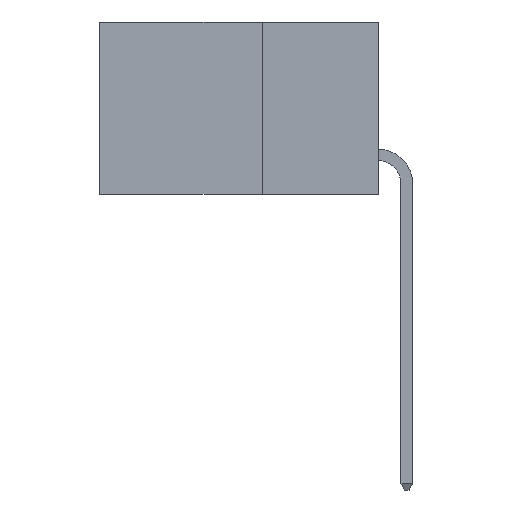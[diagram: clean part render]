
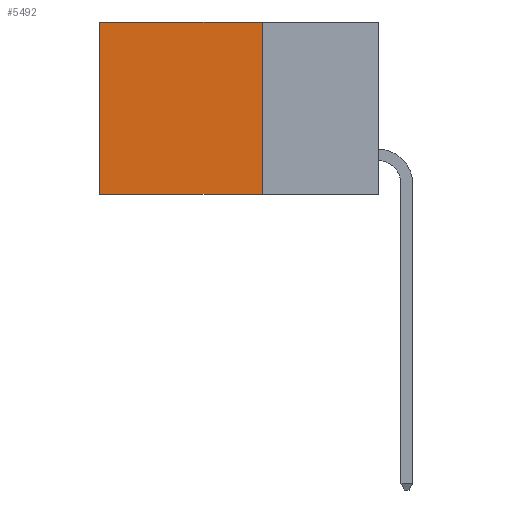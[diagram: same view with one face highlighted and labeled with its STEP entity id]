
A CAD part, left-side view. The second image highlights one B-rep face of the part: STEP entity #5492.
In plain terms, the highlighted planar face has unit normal (-1, 0, 0).
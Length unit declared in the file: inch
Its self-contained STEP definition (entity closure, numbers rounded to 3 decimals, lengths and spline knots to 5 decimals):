
#152 = PLANE ( 'NONE',  #8599 ) ;
#533 = LINE ( 'NONE', #5186, #8434 ) ;
#593 = CARTESIAN_POINT ( 'NONE',  ( 0.2615, 0.25, -0.37 ) ) ;
#1516 = VERTEX_POINT ( 'NONE', #2472 ) ;
#1662 = LINE ( 'NONE', #7751, #6808 ) ;
#1701 = CARTESIAN_POINT ( 'NONE',  ( 0.2615, 0.25, 0. ) ) ;
#1781 = VERTEX_POINT ( 'NONE', #12896 ) ;
#1804 = DIRECTION ( 'NONE',  ( 0., 0., -1. ) ) ;
#1983 = VECTOR ( 'NONE', #1804, 39.37008 ) ;
#2302 = LINE ( 'NONE', #3801, #1983 ) ;
#2472 = CARTESIAN_POINT ( 'NONE',  ( 0.2615, 0.6, -0.37 ) ) ;
#2528 = EDGE_CURVE ( 'NONE', #1781, #3534, #11298, .T. ) ;
#2982 = ORIENTED_EDGE ( 'NONE', *, *, #11586, .F. ) ;
#3303 = DIRECTION ( 'NONE',  ( 1., 0., 0. ) ) ;
#3534 = VERTEX_POINT ( 'NONE', #9424 ) ;
#3801 = CARTESIAN_POINT ( 'NONE',  ( 0.2615, 0.25, -0.37 ) ) ;
#4270 = EDGE_CURVE ( 'NONE', #9251, #1516, #1662, .T. ) ;
#4550 = ORIENTED_EDGE ( 'NONE', *, *, #4270, .F. ) ;
#5186 = CARTESIAN_POINT ( 'NONE',  ( 0.2615, 0.6, -0.37 ) ) ;
#5222 = EDGE_LOOP ( 'NONE', ( #5898, #4550, #2982, #10934 ) ) ;
#5492 = ADVANCED_FACE ( 'NONE', ( #10964 ), #152, .F. ) ;
#5898 = ORIENTED_EDGE ( 'NONE', *, *, #11180, .T. ) ;
#6808 = VECTOR ( 'NONE', #8762, 39.37008 ) ;
#7751 = CARTESIAN_POINT ( 'NONE',  ( 0.2615, 0.25, -0.37 ) ) ;
#7897 = DIRECTION ( 'NONE',  ( 0., 1., 0. ) ) ;
#8434 = VECTOR ( 'NONE', #12064, 39.37008 ) ;
#8599 = AXIS2_PLACEMENT_3D ( 'NONE', #9451, #3303, #10433 ) ;
#8762 = DIRECTION ( 'NONE',  ( 0., 1., 0. ) ) ;
#8772 = VECTOR ( 'NONE', #7897, 39.37008 ) ;
#9251 = VERTEX_POINT ( 'NONE', #593 ) ;
#9424 = CARTESIAN_POINT ( 'NONE',  ( 0.2615, 0.6, 0. ) ) ;
#9451 = CARTESIAN_POINT ( 'NONE',  ( 0.2615, 0.25, -0.37 ) ) ;
#10433 = DIRECTION ( 'NONE',  ( 0., 0., -1. ) ) ;
#10934 = ORIENTED_EDGE ( 'NONE', *, *, #2528, .T. ) ;
#10964 = FACE_OUTER_BOUND ( 'NONE', #5222, .T. ) ;
#11180 = EDGE_CURVE ( 'NONE', #3534, #1516, #533, .T. ) ;
#11298 = LINE ( 'NONE', #1701, #8772 ) ;
#11586 = EDGE_CURVE ( 'NONE', #1781, #9251, #2302, .T. ) ;
#12064 = DIRECTION ( 'NONE',  ( 0., 0., -1. ) ) ;
#12896 = CARTESIAN_POINT ( 'NONE',  ( 0.2615, 0.25, 0. ) ) ;
